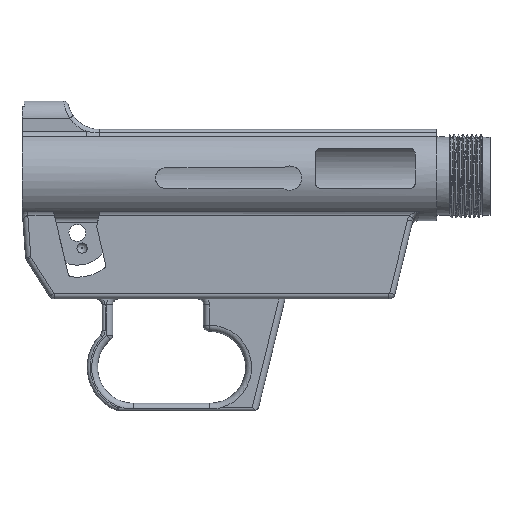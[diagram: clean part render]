
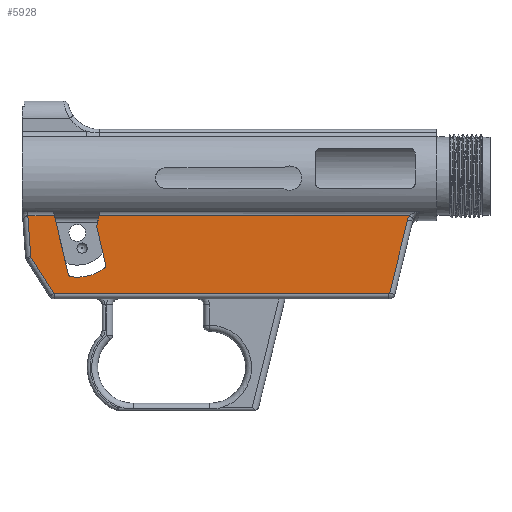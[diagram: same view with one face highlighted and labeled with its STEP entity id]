
A CAD part, left-side view. The second image highlights one B-rep face of the part: STEP entity #5928.
In plain terms, the highlighted planar face has unit normal (-1, 0, 0).
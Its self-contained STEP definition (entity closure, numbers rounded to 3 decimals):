
#82=PLANE('',#6333);
#302=FACE_OUTER_BOUND('',#643,.T.);
#643=EDGE_LOOP('',(#4112,#4113,#4114,#4115,#4116,#4117,#4118,#4119,#4120,
#4121,#4122,#4123,#4124,#4125,#4126,#4127));
#986=CIRCLE('',#6303,1.);
#988=CIRCLE('',#6307,1.);
#991=CIRCLE('',#6311,14.884);
#999=CIRCLE('',#6334,0.25);
#1000=CIRCLE('',#6335,0.25);
#1001=CIRCLE('',#6336,0.25);
#1262=B_SPLINE_CURVE_WITH_KNOTS('',3,(#9586,#9587,#9588,#9589),
 .UNSPECIFIED.,.F.,.F.,(4,4),(0.,0.148),.UNSPECIFIED.);
#1440=LINE('',#9294,#1920);
#1452=LINE('',#9333,#1932);
#1466=LINE('',#9569,#1946);
#1467=LINE('',#9572,#1947);
#1468=LINE('',#9576,#1948);
#1469=LINE('',#9580,#1949);
#1470=LINE('',#9584,#1950);
#1471=LINE('',#9591,#1951);
#1472=LINE('',#9592,#1952);
#1920=VECTOR('',#7029,10.);
#1932=VECTOR('',#7065,10.);
#1946=VECTOR('',#7109,10.);
#1947=VECTOR('',#7112,10.);
#1948=VECTOR('',#7115,10.);
#1949=VECTOR('',#7118,10.);
#1950=VECTOR('',#7121,10.);
#1951=VECTOR('',#7122,10.);
#1952=VECTOR('',#7123,10.);
#2433=VERTEX_POINT('',#9284);
#2434=VERTEX_POINT('',#9285);
#2437=VERTEX_POINT('',#9293);
#2441=VERTEX_POINT('',#9303);
#2442=VERTEX_POINT('',#9304);
#2452=VERTEX_POINT('',#9331);
#2491=VERTEX_POINT('',#9551);
#2493=VERTEX_POINT('',#9571);
#2494=VERTEX_POINT('',#9573);
#2495=VERTEX_POINT('',#9575);
#2496=VERTEX_POINT('',#9577);
#2497=VERTEX_POINT('',#9579);
#2498=VERTEX_POINT('',#9581);
#2499=VERTEX_POINT('',#9583);
#2500=VERTEX_POINT('',#9585);
#2501=VERTEX_POINT('',#9590);
#3057=EDGE_CURVE('',#2433,#2434,#986,.T.);
#3061=EDGE_CURVE('',#2437,#2434,#1440,.T.);
#3066=EDGE_CURVE('',#2441,#2442,#988,.T.);
#3071=EDGE_CURVE('',#2433,#2442,#991,.T.);
#3081=EDGE_CURVE('',#2441,#2452,#1452,.T.);
#3124=EDGE_CURVE('',#2491,#2452,#1466,.T.);
#3125=EDGE_CURVE('',#2493,#2491,#1467,.T.);
#3126=EDGE_CURVE('',#2494,#2493,#999,.T.);
#3127=EDGE_CURVE('',#2495,#2494,#1468,.T.);
#3128=EDGE_CURVE('',#2496,#2495,#1000,.T.);
#3129=EDGE_CURVE('',#2497,#2496,#1469,.T.);
#3130=EDGE_CURVE('',#2498,#2497,#1001,.T.);
#3131=EDGE_CURVE('',#2499,#2498,#1470,.T.);
#3132=EDGE_CURVE('',#2500,#2499,#1262,.T.);
#3133=EDGE_CURVE('',#2501,#2500,#1471,.T.);
#3134=EDGE_CURVE('',#2501,#2437,#1472,.T.);
#4112=ORIENTED_EDGE('',*,*,#3124,.F.);
#4113=ORIENTED_EDGE('',*,*,#3125,.F.);
#4114=ORIENTED_EDGE('',*,*,#3126,.F.);
#4115=ORIENTED_EDGE('',*,*,#3127,.F.);
#4116=ORIENTED_EDGE('',*,*,#3128,.F.);
#4117=ORIENTED_EDGE('',*,*,#3129,.F.);
#4118=ORIENTED_EDGE('',*,*,#3130,.F.);
#4119=ORIENTED_EDGE('',*,*,#3131,.F.);
#4120=ORIENTED_EDGE('',*,*,#3132,.F.);
#4121=ORIENTED_EDGE('',*,*,#3133,.F.);
#4122=ORIENTED_EDGE('',*,*,#3134,.T.);
#4123=ORIENTED_EDGE('',*,*,#3061,.T.);
#4124=ORIENTED_EDGE('',*,*,#3057,.F.);
#4125=ORIENTED_EDGE('',*,*,#3071,.T.);
#4126=ORIENTED_EDGE('',*,*,#3066,.F.);
#4127=ORIENTED_EDGE('',*,*,#3081,.T.);
#5928=ADVANCED_FACE('',(#302),#82,.T.);
#6303=AXIS2_PLACEMENT_3D('',#9286,#7021,#7022);
#6307=AXIS2_PLACEMENT_3D('',#9305,#7036,#7037);
#6311=AXIS2_PLACEMENT_3D('',#9313,#7046,#7047);
#6333=AXIS2_PLACEMENT_3D('',#9570,#7110,#7111);
#6334=AXIS2_PLACEMENT_3D('',#9574,#7113,#7114);
#6335=AXIS2_PLACEMENT_3D('',#9578,#7116,#7117);
#6336=AXIS2_PLACEMENT_3D('',#9582,#7119,#7120);
#7021=DIRECTION('center_axis',(-1.,0.,0.));
#7022=DIRECTION('ref_axis',(0.,-0.942,-0.337));
#7029=DIRECTION('',(0.,-0.225,-0.974));
#7036=DIRECTION('center_axis',(-1.,0.,0.));
#7037=DIRECTION('ref_axis',(0.,0.678,-0.735));
#7046=DIRECTION('center_axis',(1.,0.,0.));
#7047=DIRECTION('ref_axis',(0.,-1.,0.));
#7065=DIRECTION('',(0.,0.229,0.973));
#7109=DIRECTION('',(0.,-1.,0.));
#7110=DIRECTION('center_axis',(-1.,0.,0.));
#7111=DIRECTION('ref_axis',(0.,0.,1.));
#7112=DIRECTION('',(0.,0.073,0.997));
#7113=DIRECTION('center_axis',(1.,0.,0.));
#7114=DIRECTION('ref_axis',(0.,0.949,-0.315));
#7115=DIRECTION('',(0.,0.537,0.843));
#7116=DIRECTION('center_axis',(1.,0.,0.));
#7117=DIRECTION('ref_axis',(0.,0.481,-0.877));
#7118=DIRECTION('',(0.,1.,0.));
#7119=DIRECTION('center_axis',(1.,0.,0.));
#7120=DIRECTION('ref_axis',(0.,-0.992,-0.124));
#7121=DIRECTION('',(0.,0.236,-0.972));
#7122=DIRECTION('',(0.,-1.,0.));
#7123=DIRECTION('',(0.,0.225,-0.974));
#9284=CARTESIAN_POINT('',(-8.475,33.632,10.39));
#9285=CARTESIAN_POINT('',(-8.475,33.269,11.407));
#9286=CARTESIAN_POINT('Origin',(-8.475,34.243,11.182));
#9293=CARTESIAN_POINT('',(-8.475,36.258,24.36));
#9294=CARTESIAN_POINT('',(-8.475,32.672,8.823));
#9303=CARTESIAN_POINT('',(-8.475,45.771,8.217));
#9304=CARTESIAN_POINT('',(-8.475,44.947,7.458));
#9305=CARTESIAN_POINT('Origin',(-8.475,44.797,8.446));
#9313=CARTESIAN_POINT('Origin',(-8.475,42.724,22.175));
#9331=CARTESIAN_POINT('',(-8.475,50.401,27.888));
#9333=CARTESIAN_POINT('',(-8.475,43.577,-1.101));
#9551=CARTESIAN_POINT('',(-8.475,59.361,27.888));
#9569=CARTESIAN_POINT('',(-8.475,0.,27.888));
#9570=CARTESIAN_POINT('Origin',(-8.475,0.,0.));
#9571=CARTESIAN_POINT('',(-8.475,58.352,14.126));
#9572=CARTESIAN_POINT('',(-8.475,58.284,13.198));
#9573=CARTESIAN_POINT('',(-8.475,58.313,14.01));
#9574=CARTESIAN_POINT('Origin',(-8.475,58.102,14.145));
#9575=CARTESIAN_POINT('',(-8.475,50.579,1.866));
#9576=CARTESIAN_POINT('',(-8.475,46.861,-3.971));
#9577=CARTESIAN_POINT('',(-8.475,50.368,1.75));
#9578=CARTESIAN_POINT('Origin',(-8.475,50.368,2.));
#9579=CARTESIAN_POINT('',(-8.475,-61.773,1.75));
#9580=CARTESIAN_POINT('',(-8.475,0.,1.75));
#9581=CARTESIAN_POINT('',(-8.475,-62.016,1.941));
#9582=CARTESIAN_POINT('Origin',(-8.475,-61.773,2.));
#9583=CARTESIAN_POINT('',(-8.475,-67.981,26.535));
#9584=CARTESIAN_POINT('',(-8.475,-59.885,-6.843));
#9585=CARTESIAN_POINT('',(-8.475,-68.554,27.888));
#9586=CARTESIAN_POINT('Ctrl Pts',(-8.475,-68.554,27.888));
#9587=CARTESIAN_POINT('Ctrl Pts',(-8.475,-68.292,27.472));
#9588=CARTESIAN_POINT('Ctrl Pts',(-8.475,-68.097,27.013));
#9589=CARTESIAN_POINT('Ctrl Pts',(-8.475,-67.981,26.535));
#9590=CARTESIAN_POINT('',(-8.475,35.445,27.888));
#9591=CARTESIAN_POINT('',(-8.475,0.,27.888));
#9592=CARTESIAN_POINT('',(-8.475,37.307,19.808));
